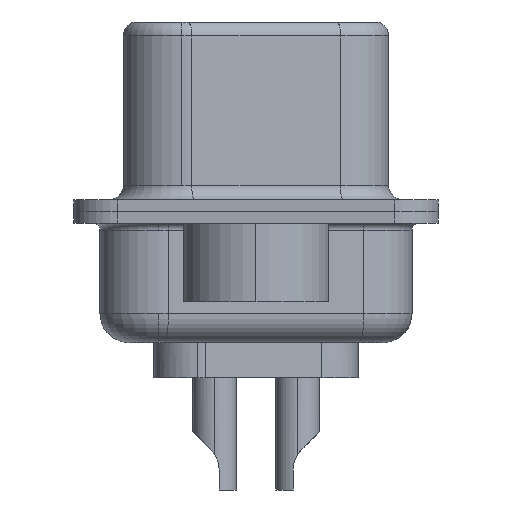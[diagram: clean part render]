
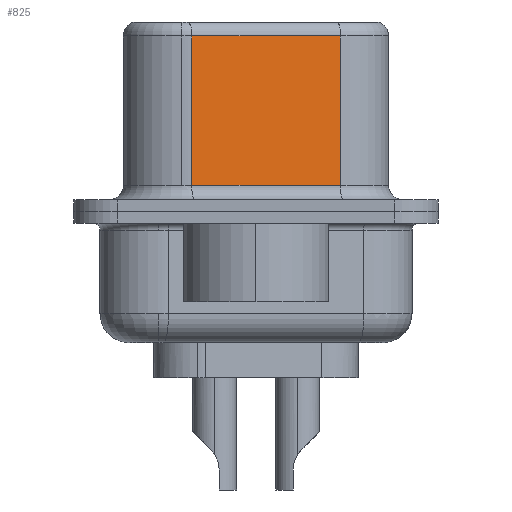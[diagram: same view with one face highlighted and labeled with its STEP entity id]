
A CAD part, left-side view. The second image highlights one B-rep face of the part: STEP entity #825.
In plain terms, the highlighted planar face has unit normal (-0.985, -0.174, 0).
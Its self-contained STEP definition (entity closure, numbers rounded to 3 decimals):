
#85 = VERTEX_POINT ( 'NONE', #19282 ) ;
#519 = VERTEX_POINT ( 'NONE', #6360 ) ;
#587 = PLANE ( 'NONE',  #20036 ) ;
#825 = ADVANCED_FACE ( 'NONE', ( #11951 ), #587, .F. ) ;
#3138 = ORIENTED_EDGE ( 'NONE', *, *, #13192, .T. ) ;
#3343 = VECTOR ( 'NONE', #11641, 1000. ) ;
#4194 = VECTOR ( 'NONE', #8637, 1000. ) ;
#5065 = LINE ( 'NONE', #7061, #16489 ) ;
#5187 = CARTESIAN_POINT ( 'NONE',  ( 4.58, -2.897, 0.9 ) ) ;
#5398 = CARTESIAN_POINT ( 'NONE',  ( 4.58, -2.897, 6.52 ) ) ;
#6360 = CARTESIAN_POINT ( 'NONE',  ( 4.58, -2.897, 6.02 ) ) ;
#6641 = EDGE_CURVE ( 'NONE', #85, #11360, #5065, .T. ) ;
#7061 = CARTESIAN_POINT ( 'NONE',  ( 3.68, 2.203, 6.52 ) ) ;
#7774 = EDGE_LOOP ( 'NONE', ( #14056, #20798, #12391, #3138 ) ) ;
#7899 = LINE ( 'NONE', #18905, #14670 ) ;
#8637 = DIRECTION ( 'NONE',  ( 0., 0., -1. ) ) ;
#10450 = LINE ( 'NONE', #18285, #4194 ) ;
#11360 = VERTEX_POINT ( 'NONE', #13989 ) ;
#11641 = DIRECTION ( 'NONE',  ( 0.174, -0.985, 0. ) ) ;
#11936 = DIRECTION ( 'NONE',  ( 0., 0., -1. ) ) ;
#11951 = FACE_OUTER_BOUND ( 'NONE', #7774, .T. ) ;
#12295 = CARTESIAN_POINT ( 'NONE',  ( 4.58, -2.897, 0.9 ) ) ;
#12391 = ORIENTED_EDGE ( 'NONE', *, *, #6641, .T. ) ;
#13192 = EDGE_CURVE ( 'NONE', #11360, #18264, #14827, .T. ) ;
#13426 = DIRECTION ( 'NONE',  ( 0.985, 0.174, 0. ) ) ;
#13641 = DIRECTION ( 'NONE',  ( -0.174, 0.985, 0. ) ) ;
#13989 = CARTESIAN_POINT ( 'NONE',  ( 3.68, 2.203, 0.9 ) ) ;
#14056 = ORIENTED_EDGE ( 'NONE', *, *, #19919, .F. ) ;
#14670 = VECTOR ( 'NONE', #19012, 1000. ) ;
#14827 = LINE ( 'NONE', #5187, #3343 ) ;
#16489 = VECTOR ( 'NONE', #11936, 1000. ) ;
#18264 = VERTEX_POINT ( 'NONE', #12295 ) ;
#18285 = CARTESIAN_POINT ( 'NONE',  ( 4.58, -2.897, 6.52 ) ) ;
#18905 = CARTESIAN_POINT ( 'NONE',  ( 4.58, -2.897, 6.02 ) ) ;
#19012 = DIRECTION ( 'NONE',  ( -0.174, 0.985, 0. ) ) ;
#19282 = CARTESIAN_POINT ( 'NONE',  ( 3.68, 2.203, 6.02 ) ) ;
#19919 = EDGE_CURVE ( 'NONE', #519, #18264, #10450, .T. ) ;
#20036 = AXIS2_PLACEMENT_3D ( 'NONE', #5398, #13426, #13641 ) ;
#20129 = EDGE_CURVE ( 'NONE', #519, #85, #7899, .T. ) ;
#20798 = ORIENTED_EDGE ( 'NONE', *, *, #20129, .T. ) ;
